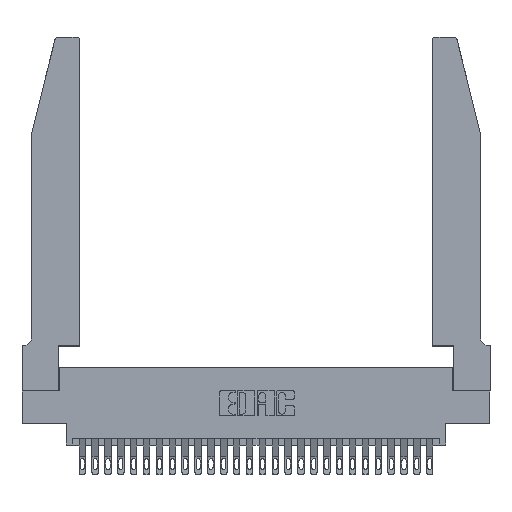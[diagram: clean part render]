
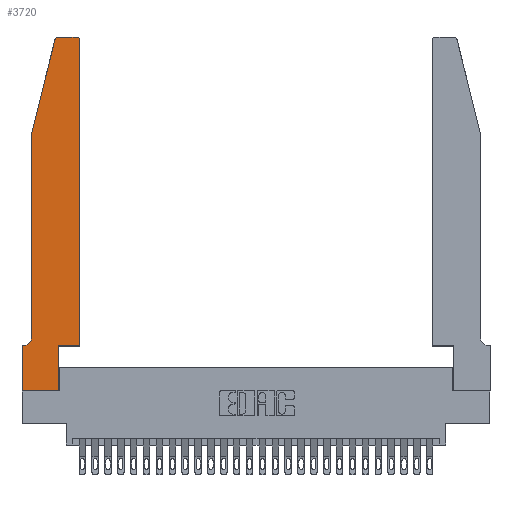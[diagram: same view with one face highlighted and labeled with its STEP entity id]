
A CAD part, top view. The second image highlights one B-rep face of the part: STEP entity #3720.
In plain terms, the highlighted planar face has unit normal (0, 0, 1).
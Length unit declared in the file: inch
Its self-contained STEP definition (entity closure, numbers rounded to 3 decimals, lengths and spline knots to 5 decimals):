
#107 = CARTESIAN_POINT ( 'NONE',  ( 0., 0., 0.37 ) ) ;
#369 = CARTESIAN_POINT ( 'NONE',  ( 0.2865, 0.35, 0.37 ) ) ;
#650 = VECTOR ( 'NONE', #16422, 39.37008 ) ;
#870 = ORIENTED_EDGE ( 'NONE', *, *, #1105, .T. ) ;
#981 = ORIENTED_EDGE ( 'NONE', *, *, #7951, .T. ) ;
#1105 = EDGE_CURVE ( 'NONE', #12011, #26962, #15140, .T. ) ;
#1439 = CARTESIAN_POINT ( 'NONE',  ( 0.2865, 0., 0.37 ) ) ;
#1531 = VERTEX_POINT ( 'NONE', #3093 ) ;
#1646 = CARTESIAN_POINT ( 'NONE',  ( 0., 0.35, 0.37 ) ) ;
#1719 = CARTESIAN_POINT ( 'NONE',  ( 0.2865, 0.35, 0.37 ) ) ;
#1722 = VECTOR ( 'NONE', #25401, 39.37008 ) ;
#2001 = DIRECTION ( 'NONE',  ( 0., 0., 1. ) ) ;
#2176 = ORIENTED_EDGE ( 'NONE', *, *, #26982, .T. ) ;
#2214 = EDGE_CURVE ( 'NONE', #20538, #6835, #16781, .T. ) ;
#2927 = EDGE_CURVE ( 'NONE', #26962, #1531, #24105, .T. ) ;
#3093 = CARTESIAN_POINT ( 'NONE',  ( 0.0055, 0.35, 0.37 ) ) ;
#3660 = LINE ( 'NONE', #20540, #9077 ) ;
#3720 = ADVANCED_FACE ( 'NONE', ( #15709 ), #13048, .T. ) ;
#3968 = DIRECTION ( 'NONE',  ( 1., 0., 0. ) ) ;
#4002 = EDGE_LOOP ( 'NONE', ( #6621, #981, #7363, #870, #20862, #28362, #27029, #2176, #7234, #15757, #27527, #24584 ) ) ;
#4251 = VECTOR ( 'NONE', #27328, 39.37008 ) ;
#5104 = CARTESIAN_POINT ( 'NONE',  ( 0.2605, 2.75, 0.37 ) ) ;
#5336 = CARTESIAN_POINT ( 'NONE',  ( 0.0755, 2., 0.37 ) ) ;
#6344 = VERTEX_POINT ( 'NONE', #24864 ) ;
#6621 = ORIENTED_EDGE ( 'NONE', *, *, #23874, .T. ) ;
#6835 = VERTEX_POINT ( 'NONE', #107 ) ;
#6989 = EDGE_CURVE ( 'NONE', #21078, #12599, #7049, .T. ) ;
#7049 = LINE ( 'NONE', #7525, #19005 ) ;
#7234 = ORIENTED_EDGE ( 'NONE', *, *, #12855, .T. ) ;
#7363 = ORIENTED_EDGE ( 'NONE', *, *, #16284, .T. ) ;
#7525 = CARTESIAN_POINT ( 'NONE',  ( 0.4505, 0.35, 0.37 ) ) ;
#7951 = EDGE_CURVE ( 'NONE', #11035, #6344, #14436, .T. ) ;
#8571 = DIRECTION ( 'NONE',  ( 0., 0., 1. ) ) ;
#9077 = VECTOR ( 'NONE', #24970, 39.37008 ) ;
#9171 = EDGE_CURVE ( 'NONE', #25515, #26275, #23741, .T. ) ;
#10183 = CARTESIAN_POINT ( 'NONE',  ( 0., 0., 0.37 ) ) ;
#10812 = VECTOR ( 'NONE', #21034, 39.37008 ) ;
#11035 = VERTEX_POINT ( 'NONE', #17188 ) ;
#11832 = CARTESIAN_POINT ( 'NONE',  ( 0.4505, 0.35, 0.37 ) ) ;
#11878 = CARTESIAN_POINT ( 'NONE',  ( 0.4505, 0.35, 0.37 ) ) ;
#11907 = VECTOR ( 'NONE', #17618, 39.37008 ) ;
#12011 = VERTEX_POINT ( 'NONE', #5336 ) ;
#12171 = CARTESIAN_POINT ( 'NONE',  ( 0.0055, 0.42, 0.37 ) ) ;
#12224 = VERTEX_POINT ( 'NONE', #1439 ) ;
#12599 = VERTEX_POINT ( 'NONE', #11832 ) ;
#12855 = EDGE_CURVE ( 'NONE', #12224, #21078, #23098, .T. ) ;
#12947 = DIRECTION ( 'NONE',  ( 0., -1., 0. ) ) ;
#13048 = PLANE ( 'NONE',  #21569 ) ;
#13888 = LINE ( 'NONE', #20977, #1722 ) ;
#13898 = CARTESIAN_POINT ( 'NONE',  ( 0.4205, 2.75, 0.37 ) ) ;
#14435 = VECTOR ( 'NONE', #12947, 39.37008 ) ;
#14436 = CIRCLE ( 'NONE', #23865, 0.03 ) ;
#14477 = DIRECTION ( 'NONE',  ( -1., 0., 0. ) ) ;
#14765 = DIRECTION ( 'NONE',  ( 1., 0., 0. ) ) ;
#15140 = LINE ( 'NONE', #16423, #14435 ) ;
#15469 = VECTOR ( 'NONE', #14765, 39.37008 ) ;
#15646 = CARTESIAN_POINT ( 'NONE',  ( 0.284, 2.72, 0.37 ) ) ;
#15709 = FACE_OUTER_BOUND ( 'NONE', #4002, .T. ) ;
#15757 = ORIENTED_EDGE ( 'NONE', *, *, #6989, .T. ) ;
#16284 = EDGE_CURVE ( 'NONE', #6344, #12011, #13888, .T. ) ;
#16422 = DIRECTION ( 'NONE',  ( 0., 1., 0. ) ) ;
#16423 = CARTESIAN_POINT ( 'NONE',  ( 0.0755, 2., 0.37 ) ) ;
#16781 = LINE ( 'NONE', #22508, #10812 ) ;
#17188 = CARTESIAN_POINT ( 'NONE',  ( 0.284, 2.75, 0.37 ) ) ;
#17556 = DIRECTION ( 'NONE',  ( 0., 0., 1. ) ) ;
#17618 = DIRECTION ( 'NONE',  ( 0., 1., 0. ) ) ;
#17890 = DIRECTION ( 'NONE',  ( 1., 0., 0. ) ) ;
#18216 = CARTESIAN_POINT ( 'NONE',  ( 0.4505, 2.72, 0.37 ) ) ;
#18804 = LINE ( 'NONE', #11878, #650 ) ;
#19005 = VECTOR ( 'NONE', #27540, 39.37008 ) ;
#20538 = VERTEX_POINT ( 'NONE', #23290 ) ;
#20540 = CARTESIAN_POINT ( 'NONE',  ( 0.0755, 0.35, 0.37 ) ) ;
#20862 = ORIENTED_EDGE ( 'NONE', *, *, #2927, .T. ) ;
#20977 = CARTESIAN_POINT ( 'NONE',  ( 0.0755, 2., 0.37 ) ) ;
#21034 = DIRECTION ( 'NONE',  ( 0., -1., 0. ) ) ;
#21078 = VERTEX_POINT ( 'NONE', #369 ) ;
#21569 = AXIS2_PLACEMENT_3D ( 'NONE', #1646, #17556, #3968 ) ;
#21576 = EDGE_CURVE ( 'NONE', #1531, #20538, #3660, .T. ) ;
#21987 = CARTESIAN_POINT ( 'NONE',  ( 0.4205, 2.72, 0.37 ) ) ;
#22508 = CARTESIAN_POINT ( 'NONE',  ( 0., 0., 0.37 ) ) ;
#22682 = AXIS2_PLACEMENT_3D ( 'NONE', #12171, #27659, #14477 ) ;
#23098 = LINE ( 'NONE', #1719, #11907 ) ;
#23290 = CARTESIAN_POINT ( 'NONE',  ( 0., 0.35, 0.37 ) ) ;
#23684 = AXIS2_PLACEMENT_3D ( 'NONE', #21987, #8571, #24200 ) ;
#23741 = CIRCLE ( 'NONE', #23684, 0.03 ) ;
#23865 = AXIS2_PLACEMENT_3D ( 'NONE', #15646, #2001, #17890 ) ;
#23874 = EDGE_CURVE ( 'NONE', #26275, #11035, #26666, .T. ) ;
#24105 = CIRCLE ( 'NONE', #22682, 0.07 ) ;
#24200 = DIRECTION ( 'NONE',  ( 1., 0., 0. ) ) ;
#24584 = ORIENTED_EDGE ( 'NONE', *, *, #9171, .T. ) ;
#24864 = CARTESIAN_POINT ( 'NONE',  ( 0.25487, 2.72718, 0.37 ) ) ;
#24970 = DIRECTION ( 'NONE',  ( -1., 0., 0. ) ) ;
#25401 = DIRECTION ( 'NONE',  ( -0.239, -0.971, 0. ) ) ;
#25515 = VERTEX_POINT ( 'NONE', #18216 ) ;
#25772 = CARTESIAN_POINT ( 'NONE',  ( 0.0755, 0.42, 0.37 ) ) ;
#26275 = VERTEX_POINT ( 'NONE', #13898 ) ;
#26666 = LINE ( 'NONE', #5104, #4251 ) ;
#26772 = EDGE_CURVE ( 'NONE', #12599, #25515, #18804, .T. ) ;
#26962 = VERTEX_POINT ( 'NONE', #25772 ) ;
#26982 = EDGE_CURVE ( 'NONE', #6835, #12224, #27183, .T. ) ;
#27029 = ORIENTED_EDGE ( 'NONE', *, *, #2214, .T. ) ;
#27183 = LINE ( 'NONE', #10183, #15469 ) ;
#27328 = DIRECTION ( 'NONE',  ( -1., 0., 0. ) ) ;
#27527 = ORIENTED_EDGE ( 'NONE', *, *, #26772, .T. ) ;
#27540 = DIRECTION ( 'NONE',  ( 1., 0., 0. ) ) ;
#27659 = DIRECTION ( 'NONE',  ( 0., 0., -1. ) ) ;
#28362 = ORIENTED_EDGE ( 'NONE', *, *, #21576, .T. ) ;
